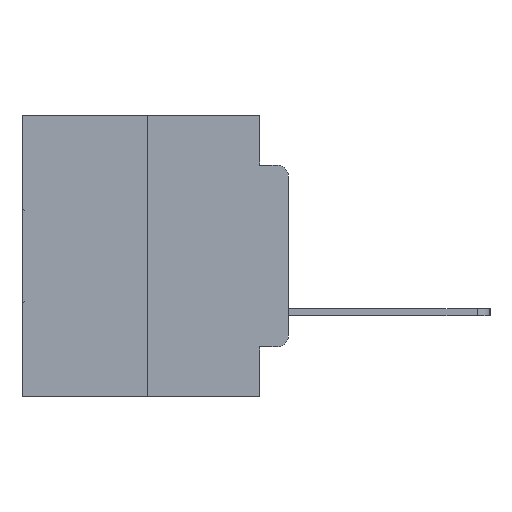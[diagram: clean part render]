
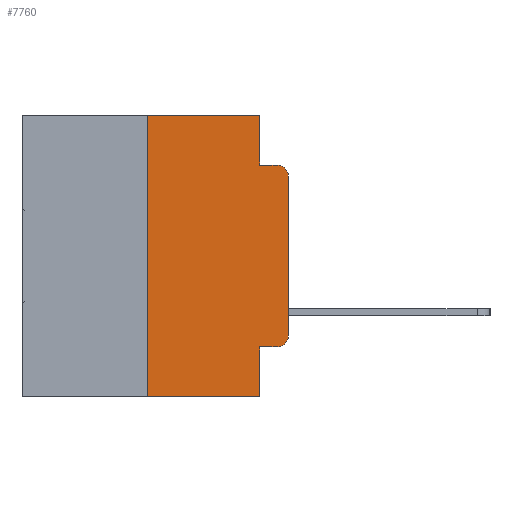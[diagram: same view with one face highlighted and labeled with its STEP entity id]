
A CAD part, left-side view. The second image highlights one B-rep face of the part: STEP entity #7760.
In plain terms, the highlighted planar face has unit normal (-1, 0, 0).
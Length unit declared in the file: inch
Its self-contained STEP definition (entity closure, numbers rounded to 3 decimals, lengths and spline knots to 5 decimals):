
#59 = ORIENTED_EDGE ( 'NONE', *, *, #22132, .F. ) ;
#88 = ORIENTED_EDGE ( 'NONE', *, *, #1167, .T. ) ;
#189 = ORIENTED_EDGE ( 'NONE', *, *, #28823, .T. ) ;
#361 = ORIENTED_EDGE ( 'NONE', *, *, #30064, .T. ) ;
#507 = CARTESIAN_POINT ( 'NONE',  ( 0., 0.051, 0. ) ) ;
#824 = VERTEX_POINT ( 'NONE', #23503 ) ;
#851 = CARTESIAN_POINT ( 'NONE',  ( 0., 0.02, -0.4115 ) ) ;
#881 = AXIS2_PLACEMENT_3D ( 'NONE', #1838, #18871, #4459 ) ;
#971 = VERTEX_POINT ( 'NONE', #16278 ) ;
#1125 = ORIENTED_EDGE ( 'NONE', *, *, #19390, .F. ) ;
#1167 = EDGE_CURVE ( 'NONE', #6954, #3272, #22125, .T. ) ;
#1838 = CARTESIAN_POINT ( 'NONE',  ( 0., 0.02, -0.3915 ) ) ;
#3016 = VECTOR ( 'NONE', #20610, 39.37008 ) ;
#3272 = VERTEX_POINT ( 'NONE', #851 ) ;
#3380 = ORIENTED_EDGE ( 'NONE', *, *, #8100, .F. ) ;
#3813 = ORIENTED_EDGE ( 'NONE', *, *, #26596, .F. ) ;
#3946 = VECTOR ( 'NONE', #23182, 39.37008 ) ;
#4459 = DIRECTION ( 'NONE',  ( 0., 0., -1. ) ) ;
#4594 = EDGE_CURVE ( 'NONE', #6954, #24307, #29736, .T. ) ;
#4777 = FACE_OUTER_BOUND ( 'NONE', #13677, .T. ) ;
#5209 = ORIENTED_EDGE ( 'NONE', *, *, #5732, .T. ) ;
#5302 = VERTEX_POINT ( 'NONE', #25977 ) ;
#5732 = EDGE_CURVE ( 'NONE', #971, #27357, #28965, .T. ) ;
#6954 = VERTEX_POINT ( 'NONE', #7620 ) ;
#7080 = ORIENTED_EDGE ( 'NONE', *, *, #7433, .T. ) ;
#7306 = ORIENTED_EDGE ( 'NONE', *, *, #4594, .F. ) ;
#7433 = EDGE_CURVE ( 'NONE', #824, #971, #27451, .T. ) ;
#7620 = CARTESIAN_POINT ( 'NONE',  ( 0., 0.051, -0.4115 ) ) ;
#7760 = ADVANCED_FACE ( 'NONE', ( #4777 ), #9816, .F. ) ;
#8100 = EDGE_CURVE ( 'NONE', #27833, #24350, #28775, .T. ) ;
#9291 = CARTESIAN_POINT ( 'NONE',  ( 0., 0.473, 0. ) ) ;
#9816 = PLANE ( 'NONE',  #25829 ) ;
#10323 = CARTESIAN_POINT ( 'NONE',  ( 0., 0., 0. ) ) ;
#10546 = CARTESIAN_POINT ( 'NONE',  ( 0., 0.473, -0.5 ) ) ;
#11113 = DIRECTION ( 'NONE',  ( 0., 0., -1. ) ) ;
#11295 = CARTESIAN_POINT ( 'NONE',  ( 0., 0.051, 0. ) ) ;
#11302 = DIRECTION ( 'NONE',  ( -1., 0., 0. ) ) ;
#11381 = DIRECTION ( 'NONE',  ( 0., 0., 1. ) ) ;
#11918 = VECTOR ( 'NONE', #28657, 39.37008 ) ;
#12221 = DIRECTION ( 'NONE',  ( 1., 0., 0. ) ) ;
#13677 = EDGE_LOOP ( 'NONE', ( #7080, #5209, #3813, #59, #1125, #3380, #189, #7306, #88, #361 ) ) ;
#14063 = DIRECTION ( 'NONE',  ( 0., -1., 0. ) ) ;
#15424 = CARTESIAN_POINT ( 'NONE',  ( 0., 0.051, 0. ) ) ;
#16278 = CARTESIAN_POINT ( 'NONE',  ( 0., 0., -0.1085 ) ) ;
#16427 = DIRECTION ( 'NONE',  ( 0., 0., -1. ) ) ;
#18871 = DIRECTION ( 'NONE',  ( -1., 0., 0. ) ) ;
#19061 = CIRCLE ( 'NONE', #881, 0.02 ) ;
#19334 = VECTOR ( 'NONE', #16427, 39.37008 ) ;
#19390 = EDGE_CURVE ( 'NONE', #24350, #20914, #22221, .T. ) ;
#19532 = CARTESIAN_POINT ( 'NONE',  ( 0., 0.051, -0.5 ) ) ;
#19615 = AXIS2_PLACEMENT_3D ( 'NONE', #24903, #11302, #11113 ) ;
#19881 = VECTOR ( 'NONE', #29346, 39.37008 ) ;
#20014 = VECTOR ( 'NONE', #14063, 39.37008 ) ;
#20566 = CARTESIAN_POINT ( 'NONE',  ( 0., 0.25, 0. ) ) ;
#20575 = LINE ( 'NONE', #11295, #19881 ) ;
#20576 = CARTESIAN_POINT ( 'NONE',  ( 0., 0.051, -0.4115 ) ) ;
#20610 = DIRECTION ( 'NONE',  ( 0., -1., 0. ) ) ;
#20705 = LINE ( 'NONE', #25358, #20014 ) ;
#20914 = VERTEX_POINT ( 'NONE', #507 ) ;
#21561 = CARTESIAN_POINT ( 'NONE',  ( 0., 0.25, -0.5 ) ) ;
#21564 = VECTOR ( 'NONE', #24036, 39.37008 ) ;
#22125 = LINE ( 'NONE', #20576, #3016 ) ;
#22132 = EDGE_CURVE ( 'NONE', #20914, #5302, #20575, .T. ) ;
#22221 = LINE ( 'NONE', #9291, #3946 ) ;
#22885 = VECTOR ( 'NONE', #11381, 39.37008 ) ;
#23182 = DIRECTION ( 'NONE',  ( 0., -1., 0. ) ) ;
#23503 = CARTESIAN_POINT ( 'NONE',  ( 0., 0., -0.3915 ) ) ;
#24036 = DIRECTION ( 'NONE',  ( 0., 0., 1. ) ) ;
#24307 = VERTEX_POINT ( 'NONE', #19532 ) ;
#24350 = VERTEX_POINT ( 'NONE', #28325 ) ;
#24903 = CARTESIAN_POINT ( 'NONE',  ( 0., 0.02, -0.1085 ) ) ;
#25358 = CARTESIAN_POINT ( 'NONE',  ( 0., 0.051, -0.0885 ) ) ;
#25809 = CARTESIAN_POINT ( 'NONE',  ( 0., 0.473, 0. ) ) ;
#25829 = AXIS2_PLACEMENT_3D ( 'NONE', #25809, #12221, #28002 ) ;
#25977 = CARTESIAN_POINT ( 'NONE',  ( 0., 0.051, -0.0885 ) ) ;
#26596 = EDGE_CURVE ( 'NONE', #5302, #27357, #20705, .T. ) ;
#27357 = VERTEX_POINT ( 'NONE', #28712 ) ;
#27451 = LINE ( 'NONE', #10323, #21564 ) ;
#27833 = VERTEX_POINT ( 'NONE', #21561 ) ;
#28002 = DIRECTION ( 'NONE',  ( 0., 0., -1. ) ) ;
#28325 = CARTESIAN_POINT ( 'NONE',  ( 0., 0.25, 0. ) ) ;
#28657 = DIRECTION ( 'NONE',  ( 0., -1., 0. ) ) ;
#28712 = CARTESIAN_POINT ( 'NONE',  ( 0., 0.02, -0.0885 ) ) ;
#28775 = LINE ( 'NONE', #20566, #22885 ) ;
#28823 = EDGE_CURVE ( 'NONE', #27833, #24307, #29903, .T. ) ;
#28965 = CIRCLE ( 'NONE', #19615, 0.02 ) ;
#29346 = DIRECTION ( 'NONE',  ( 0., 0., -1. ) ) ;
#29736 = LINE ( 'NONE', #15424, #19334 ) ;
#29903 = LINE ( 'NONE', #10546, #11918 ) ;
#30064 = EDGE_CURVE ( 'NONE', #3272, #824, #19061, .T. ) ;
